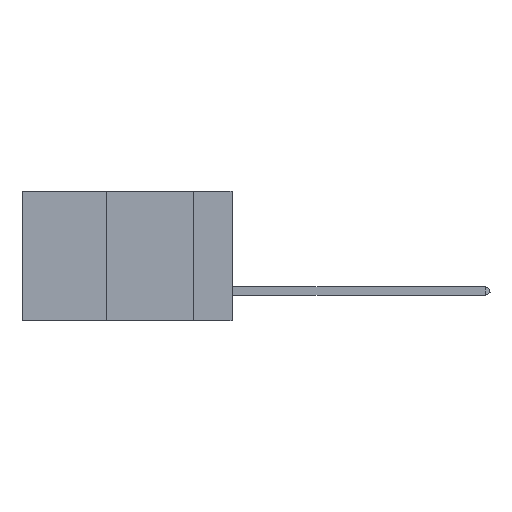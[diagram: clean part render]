
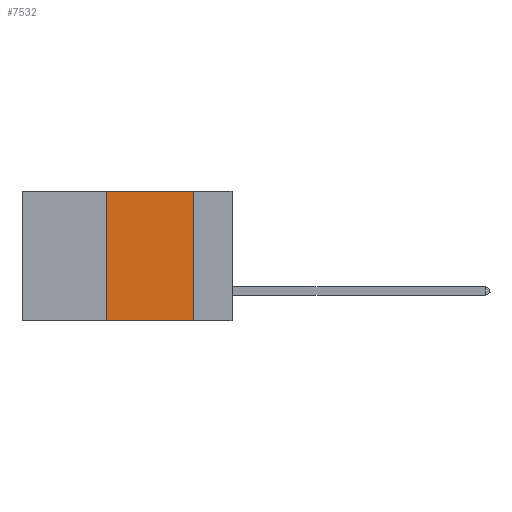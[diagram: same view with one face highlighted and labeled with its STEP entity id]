
A CAD part, left-side view. The second image highlights one B-rep face of the part: STEP entity #7532.
In plain terms, the highlighted planar face has unit normal (-1, 0, 0).
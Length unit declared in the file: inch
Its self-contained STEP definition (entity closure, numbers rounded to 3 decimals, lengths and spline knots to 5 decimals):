
#667 = VECTOR ( 'NONE', #18008, 39.37008 ) ;
#2651 = ORIENTED_EDGE ( 'NONE', *, *, #9180, .T. ) ;
#2825 = ORIENTED_EDGE ( 'NONE', *, *, #10905, .F. ) ;
#3225 = CARTESIAN_POINT ( 'NONE',  ( 0., 0.6, -0.37 ) ) ;
#3664 = CARTESIAN_POINT ( 'NONE',  ( 0., 0.11, -0.37 ) ) ;
#5040 = EDGE_CURVE ( 'NONE', #16995, #5428, #11535, .T. ) ;
#5136 = DIRECTION ( 'NONE',  ( 1., 0., 0. ) ) ;
#5428 = VERTEX_POINT ( 'NONE', #17500 ) ;
#5743 = LINE ( 'NONE', #10240, #6905 ) ;
#5855 = CARTESIAN_POINT ( 'NONE',  ( 0., 0.36, 0. ) ) ;
#5931 = FACE_OUTER_BOUND ( 'NONE', #13136, .T. ) ;
#6238 = DIRECTION ( 'NONE',  ( 0., -1., 0. ) ) ;
#6786 = CARTESIAN_POINT ( 'NONE',  ( 0., 0.11, 0. ) ) ;
#6905 = VECTOR ( 'NONE', #19271, 39.37008 ) ;
#7427 = LINE ( 'NONE', #12211, #13312 ) ;
#7532 = ADVANCED_FACE ( 'NONE', ( #5931 ), #18593, .F. ) ;
#9180 = EDGE_CURVE ( 'NONE', #16995, #10756, #16833, .T. ) ;
#9467 = ORIENTED_EDGE ( 'NONE', *, *, #12194, .F. ) ;
#10240 = CARTESIAN_POINT ( 'NONE',  ( 0., 0.6, 0. ) ) ;
#10756 = VERTEX_POINT ( 'NONE', #3664 ) ;
#10905 = EDGE_CURVE ( 'NONE', #18363, #10756, #7427, .T. ) ;
#11127 = DIRECTION ( 'NONE',  ( 0., 0., -1. ) ) ;
#11535 = LINE ( 'NONE', #5855, #667 ) ;
#11989 = VECTOR ( 'NONE', #6238, 39.37008 ) ;
#12194 = EDGE_CURVE ( 'NONE', #5428, #18363, #5743, .T. ) ;
#12211 = CARTESIAN_POINT ( 'NONE',  ( 0., 0.11, 0. ) ) ;
#13136 = EDGE_LOOP ( 'NONE', ( #2825, #9467, #15014, #2651 ) ) ;
#13312 = VECTOR ( 'NONE', #13829, 39.37008 ) ;
#13829 = DIRECTION ( 'NONE',  ( 0., 0., -1. ) ) ;
#14123 = CARTESIAN_POINT ( 'NONE',  ( 0., 0.6, 0. ) ) ;
#15014 = ORIENTED_EDGE ( 'NONE', *, *, #5040, .F. ) ;
#16833 = LINE ( 'NONE', #3225, #11989 ) ;
#16901 = AXIS2_PLACEMENT_3D ( 'NONE', #14123, #5136, #11127 ) ;
#16995 = VERTEX_POINT ( 'NONE', #18002 ) ;
#17500 = CARTESIAN_POINT ( 'NONE',  ( 0., 0.36, 0. ) ) ;
#18002 = CARTESIAN_POINT ( 'NONE',  ( 0., 0.36, -0.37 ) ) ;
#18008 = DIRECTION ( 'NONE',  ( 0., 0., 1. ) ) ;
#18363 = VERTEX_POINT ( 'NONE', #6786 ) ;
#18593 = PLANE ( 'NONE',  #16901 ) ;
#19271 = DIRECTION ( 'NONE',  ( 0., -1., 0. ) ) ;
